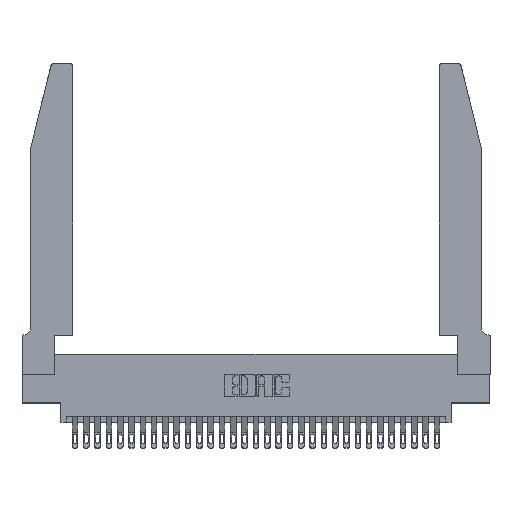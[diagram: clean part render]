
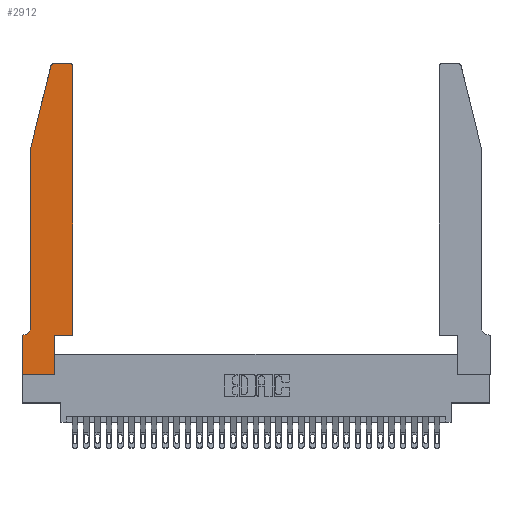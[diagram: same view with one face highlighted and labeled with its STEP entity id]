
A CAD part, top view. The second image highlights one B-rep face of the part: STEP entity #2912.
In plain terms, the highlighted planar face has unit normal (0, 0, 1).
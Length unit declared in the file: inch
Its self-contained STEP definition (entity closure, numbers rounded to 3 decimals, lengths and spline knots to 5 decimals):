
#154 = CARTESIAN_POINT ( 'NONE',  ( 0.2865, 0.35, 0.37 ) ) ;
#591 = ORIENTED_EDGE ( 'NONE', *, *, #5458, .T. ) ;
#644 = DIRECTION ( 'NONE',  ( 0., 0., 1. ) ) ;
#873 = EDGE_CURVE ( 'NONE', #20554, #25905, #14749, .T. ) ;
#1148 = EDGE_CURVE ( 'NONE', #4109, #28384, #30354, .T. ) ;
#1289 = ORIENTED_EDGE ( 'NONE', *, *, #27245, .T. ) ;
#2055 = EDGE_CURVE ( 'NONE', #4760, #16087, #21258, .T. ) ;
#2102 = DIRECTION ( 'NONE',  ( -1., 0., 0. ) ) ;
#2346 = CARTESIAN_POINT ( 'NONE',  ( 0., 0., 0.37 ) ) ;
#2912 = ADVANCED_FACE ( 'NONE', ( #12593 ), #14629, .T. ) ;
#2950 = AXIS2_PLACEMENT_3D ( 'NONE', #4559, #22465, #2102 ) ;
#3226 = CARTESIAN_POINT ( 'NONE',  ( 0.0755, 2., 0.37 ) ) ;
#3480 = VECTOR ( 'NONE', #16924, 39.37008 ) ;
#3804 = VECTOR ( 'NONE', #8008, 39.37008 ) ;
#4109 = VERTEX_POINT ( 'NONE', #16913 ) ;
#4334 = VERTEX_POINT ( 'NONE', #154 ) ;
#4530 = CARTESIAN_POINT ( 'NONE',  ( 0.0755, 0.42, 0.37 ) ) ;
#4559 = CARTESIAN_POINT ( 'NONE',  ( 0.0055, 0.42, 0.37 ) ) ;
#4715 = EDGE_CURVE ( 'NONE', #6735, #4109, #13260, .T. ) ;
#4760 = VERTEX_POINT ( 'NONE', #13955 ) ;
#4782 = VERTEX_POINT ( 'NONE', #28882 ) ;
#5192 = AXIS2_PLACEMENT_3D ( 'NONE', #30393, #644, #29436 ) ;
#5458 = EDGE_CURVE ( 'NONE', #4334, #14525, #11751, .T. ) ;
#5864 = CIRCLE ( 'NONE', #5192, 0.03 ) ;
#6735 = VERTEX_POINT ( 'NONE', #4530 ) ;
#7791 = LINE ( 'NONE', #2346, #3480 ) ;
#7810 = ORIENTED_EDGE ( 'NONE', *, *, #18384, .T. ) ;
#8008 = DIRECTION ( 'NONE',  ( -1., 0., 0. ) ) ;
#8117 = VECTOR ( 'NONE', #15840, 39.37008 ) ;
#9161 = DIRECTION ( 'NONE',  ( 0., 0., 1. ) ) ;
#9169 = CARTESIAN_POINT ( 'NONE',  ( 0.0755, 2., 0.37 ) ) ;
#9440 = ORIENTED_EDGE ( 'NONE', *, *, #873, .T. ) ;
#9523 = CARTESIAN_POINT ( 'NONE',  ( 0., 0., 0.37 ) ) ;
#9842 = AXIS2_PLACEMENT_3D ( 'NONE', #29813, #9161, #15304 ) ;
#10203 = EDGE_CURVE ( 'NONE', #25905, #4760, #5864, .T. ) ;
#10228 = VERTEX_POINT ( 'NONE', #24565 ) ;
#11211 = LINE ( 'NONE', #20460, #22617 ) ;
#11620 = VECTOR ( 'NONE', #28786, 39.37008 ) ;
#11750 = DIRECTION ( 'NONE',  ( 1., 0., 0. ) ) ;
#11751 = LINE ( 'NONE', #20935, #12471 ) ;
#11769 = CARTESIAN_POINT ( 'NONE',  ( 0., 0.35, 0.37 ) ) ;
#11888 = CARTESIAN_POINT ( 'NONE',  ( 0.4205, 2.75, 0.37 ) ) ;
#11998 = DIRECTION ( 'NONE',  ( 0., -1., 0. ) ) ;
#12471 = VECTOR ( 'NONE', #25858, 39.37008 ) ;
#12593 = FACE_OUTER_BOUND ( 'NONE', #14632, .T. ) ;
#12700 = CARTESIAN_POINT ( 'NONE',  ( 0.284, 2.75, 0.37 ) ) ;
#12748 = CARTESIAN_POINT ( 'NONE',  ( 0.4505, 0.35, 0.37 ) ) ;
#13074 = EDGE_CURVE ( 'NONE', #4782, #20554, #15492, .T. ) ;
#13260 = CIRCLE ( 'NONE', #2950, 0.07 ) ;
#13695 = VERTEX_POINT ( 'NONE', #9523 ) ;
#13955 = CARTESIAN_POINT ( 'NONE',  ( 0.25487, 2.72718, 0.37 ) ) ;
#14438 = ORIENTED_EDGE ( 'NONE', *, *, #4715, .T. ) ;
#14525 = VERTEX_POINT ( 'NONE', #12748 ) ;
#14629 = PLANE ( 'NONE',  #9842 ) ;
#14632 = EDGE_LOOP ( 'NONE', ( #9440, #24965, #17618, #7810, #14438, #28744, #21740, #1289, #14884, #591, #29737, #15011 ) ) ;
#14749 = LINE ( 'NONE', #25684, #8117 ) ;
#14884 = ORIENTED_EDGE ( 'NONE', *, *, #29980, .T. ) ;
#15011 = ORIENTED_EDGE ( 'NONE', *, *, #13074, .T. ) ;
#15304 = DIRECTION ( 'NONE',  ( 1., 0., 0. ) ) ;
#15492 = CIRCLE ( 'NONE', #31962, 0.03 ) ;
#15778 = EDGE_CURVE ( 'NONE', #14525, #4782, #11211, .T. ) ;
#15840 = DIRECTION ( 'NONE',  ( -1., 0., 0. ) ) ;
#16050 = CARTESIAN_POINT ( 'NONE',  ( 0.0755, 2., 0.37 ) ) ;
#16087 = VERTEX_POINT ( 'NONE', #9169 ) ;
#16913 = CARTESIAN_POINT ( 'NONE',  ( 0.0055, 0.35, 0.37 ) ) ;
#16924 = DIRECTION ( 'NONE',  ( 1., 0., 0. ) ) ;
#16927 = DIRECTION ( 'NONE',  ( 0., 0., 1. ) ) ;
#17028 = CARTESIAN_POINT ( 'NONE',  ( 0.4205, 2.72, 0.37 ) ) ;
#17527 = LINE ( 'NONE', #21206, #11620 ) ;
#17618 = ORIENTED_EDGE ( 'NONE', *, *, #2055, .T. ) ;
#18218 = DIRECTION ( 'NONE',  ( 0., -1., 0. ) ) ;
#18355 = DIRECTION ( 'NONE',  ( -0.239, -0.971, 0. ) ) ;
#18384 = EDGE_CURVE ( 'NONE', #16087, #6735, #26769, .T. ) ;
#19313 = VECTOR ( 'NONE', #18355, 39.37008 ) ;
#20460 = CARTESIAN_POINT ( 'NONE',  ( 0.4505, 0.35, 0.37 ) ) ;
#20481 = CARTESIAN_POINT ( 'NONE',  ( 0.0755, 0.35, 0.37 ) ) ;
#20554 = VERTEX_POINT ( 'NONE', #11888 ) ;
#20935 = CARTESIAN_POINT ( 'NONE',  ( 0.4505, 0.35, 0.37 ) ) ;
#21206 = CARTESIAN_POINT ( 'NONE',  ( 0.2865, 0.35, 0.37 ) ) ;
#21258 = LINE ( 'NONE', #16050, #19313 ) ;
#21534 = CARTESIAN_POINT ( 'NONE',  ( 0., 0., 0.37 ) ) ;
#21740 = ORIENTED_EDGE ( 'NONE', *, *, #30224, .T. ) ;
#21816 = VECTOR ( 'NONE', #11998, 39.37008 ) ;
#22465 = DIRECTION ( 'NONE',  ( 0., 0., -1. ) ) ;
#22617 = VECTOR ( 'NONE', #23410, 39.37008 ) ;
#23410 = DIRECTION ( 'NONE',  ( 0., 1., 0. ) ) ;
#24565 = CARTESIAN_POINT ( 'NONE',  ( 0.2865, 0., 0.37 ) ) ;
#24965 = ORIENTED_EDGE ( 'NONE', *, *, #10203, .T. ) ;
#25684 = CARTESIAN_POINT ( 'NONE',  ( 0.2605, 2.75, 0.37 ) ) ;
#25858 = DIRECTION ( 'NONE',  ( 1., 0., 0. ) ) ;
#25905 = VERTEX_POINT ( 'NONE', #12700 ) ;
#26501 = LINE ( 'NONE', #21534, #21816 ) ;
#26769 = LINE ( 'NONE', #3226, #32203 ) ;
#27245 = EDGE_CURVE ( 'NONE', #13695, #10228, #7791, .T. ) ;
#28384 = VERTEX_POINT ( 'NONE', #11769 ) ;
#28744 = ORIENTED_EDGE ( 'NONE', *, *, #1148, .T. ) ;
#28786 = DIRECTION ( 'NONE',  ( 0., 1., 0. ) ) ;
#28882 = CARTESIAN_POINT ( 'NONE',  ( 0.4505, 2.72, 0.37 ) ) ;
#29436 = DIRECTION ( 'NONE',  ( 1., 0., 0. ) ) ;
#29737 = ORIENTED_EDGE ( 'NONE', *, *, #15778, .T. ) ;
#29813 = CARTESIAN_POINT ( 'NONE',  ( 0., 0.35, 0.37 ) ) ;
#29980 = EDGE_CURVE ( 'NONE', #10228, #4334, #17527, .T. ) ;
#30224 = EDGE_CURVE ( 'NONE', #28384, #13695, #26501, .T. ) ;
#30354 = LINE ( 'NONE', #20481, #3804 ) ;
#30393 = CARTESIAN_POINT ( 'NONE',  ( 0.284, 2.72, 0.37 ) ) ;
#31962 = AXIS2_PLACEMENT_3D ( 'NONE', #17028, #16927, #11750 ) ;
#32203 = VECTOR ( 'NONE', #18218, 39.37008 ) ;
